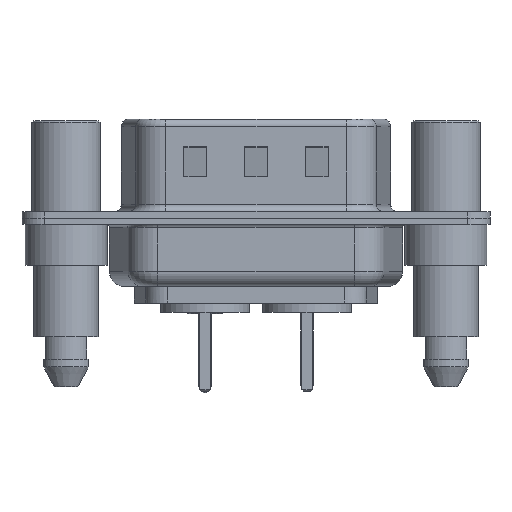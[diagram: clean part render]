
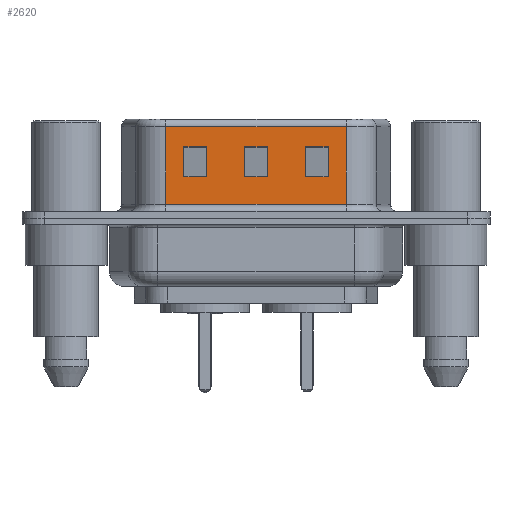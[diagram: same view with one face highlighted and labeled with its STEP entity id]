
A CAD part, front view. The second image highlights one B-rep face of the part: STEP entity #2620.
In plain terms, the highlighted planar face has unit normal (0, -1, 0).
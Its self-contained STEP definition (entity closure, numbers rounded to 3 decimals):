
#132 = LINE ( 'NONE', #7916, #21439 ) ;
#364 = DIRECTION ( 'NONE',  ( -1., 0., 0. ) ) ;
#538 = CARTESIAN_POINT ( 'NONE',  ( 18.45, -4.58, 0.9 ) ) ;
#800 = DIRECTION ( 'NONE',  ( -1., 0., 0. ) ) ;
#805 = DIRECTION ( 'NONE',  ( 0., 0., 1. ) ) ;
#951 = ORIENTED_EDGE ( 'NONE', *, *, #12862, .T. ) ;
#1283 = EDGE_LOOP ( 'NONE', ( #7963, #20948, #951, #21073 ) ) ;
#1383 = CARTESIAN_POINT ( 'NONE',  ( 7.75, -4.58, 4.705 ) ) ;
#1507 = VECTOR ( 'NONE', #8940, 1000. ) ;
#1517 = EDGE_CURVE ( 'NONE', #7936, #8701, #11608, .T. ) ;
#1711 = CARTESIAN_POINT ( 'NONE',  ( 9.25, -4.58, 6.52 ) ) ;
#2431 = VERTEX_POINT ( 'NONE', #6378 ) ;
#2462 = CARTESIAN_POINT ( 'NONE',  ( 17.25, -4.58, 4.705 ) ) ;
#2620 = ADVANCED_FACE ( 'NONE', ( #16115, #3143, #2628, #20034 ), #4380, .F. ) ;
#2628 = FACE_BOUND ( 'NONE', #5659, .T. ) ;
#2681 = CARTESIAN_POINT ( 'NONE',  ( 18.45, -4.58, 6.52 ) ) ;
#2894 = ORIENTED_EDGE ( 'NONE', *, *, #5573, .T. ) ;
#3143 = FACE_BOUND ( 'NONE', #11406, .T. ) ;
#3395 = ORIENTED_EDGE ( 'NONE', *, *, #7522, .T. ) ;
#3493 = VECTOR ( 'NONE', #6752, 1000. ) ;
#3592 = ORIENTED_EDGE ( 'NONE', *, *, #9536, .T. ) ;
#3833 = CARTESIAN_POINT ( 'NONE',  ( 22.45, -4.58, 4.705 ) ) ;
#4087 = VERTEX_POINT ( 'NONE', #10236 ) ;
#4175 = ORIENTED_EDGE ( 'NONE', *, *, #19616, .T. ) ;
#4380 = PLANE ( 'NONE',  #20349 ) ;
#4591 = VECTOR ( 'NONE', #17236, 1000. ) ;
#4650 = CARTESIAN_POINT ( 'NONE',  ( 15.75, -4.58, 4.705 ) ) ;
#4708 = LINE ( 'NONE', #6751, #13131 ) ;
#4723 = CARTESIAN_POINT ( 'NONE',  ( 7.75, -4.58, 6.52 ) ) ;
#4908 = ORIENTED_EDGE ( 'NONE', *, *, #15381, .T. ) ;
#5039 = VERTEX_POINT ( 'NONE', #21277 ) ;
#5105 = VERTEX_POINT ( 'NONE', #6813 ) ;
#5573 = EDGE_CURVE ( 'NONE', #10613, #7936, #10167, .T. ) ;
#5659 = EDGE_LOOP ( 'NONE', ( #14795, #10542, #4175, #13485 ) ) ;
#5713 = VECTOR ( 'NONE', #21201, 1000. ) ;
#5733 = DIRECTION ( 'NONE',  ( 1., 0., 0. ) ) ;
#5799 = LINE ( 'NONE', #20135, #14294 ) ;
#5944 = LINE ( 'NONE', #15727, #1507 ) ;
#6378 = CARTESIAN_POINT ( 'NONE',  ( 11.75, -4.58, 2.705 ) ) ;
#6681 = DIRECTION ( 'NONE',  ( 0., 0., -1. ) ) ;
#6751 = CARTESIAN_POINT ( 'NONE',  ( 13.25, -4.58, 6.52 ) ) ;
#6752 = DIRECTION ( 'NONE',  ( 0., 0., -1. ) ) ;
#6813 = CARTESIAN_POINT ( 'NONE',  ( 6.55, -4.58, 0.9 ) ) ;
#7059 = CARTESIAN_POINT ( 'NONE',  ( 11.75, -4.58, 6.52 ) ) ;
#7217 = VERTEX_POINT ( 'NONE', #538 ) ;
#7449 = EDGE_CURVE ( 'NONE', #5105, #7217, #132, .T. ) ;
#7522 = EDGE_CURVE ( 'NONE', #17392, #8755, #20394, .T. ) ;
#7586 = CARTESIAN_POINT ( 'NONE',  ( 18.45, -4.58, 6.52 ) ) ;
#7704 = DIRECTION ( 'NONE',  ( 1., 0., 0. ) ) ;
#7743 = DIRECTION ( 'NONE',  ( 0., 0., 1. ) ) ;
#7916 = CARTESIAN_POINT ( 'NONE',  ( 18.45, -4.58, 0.9 ) ) ;
#7936 = VERTEX_POINT ( 'NONE', #2462 ) ;
#7954 = LINE ( 'NONE', #1711, #3493 ) ;
#7963 = ORIENTED_EDGE ( 'NONE', *, *, #12365, .F. ) ;
#7995 = VECTOR ( 'NONE', #14859, 1000. ) ;
#8302 = VECTOR ( 'NONE', #7704, 1000. ) ;
#8466 = LINE ( 'NONE', #12456, #17493 ) ;
#8701 = VERTEX_POINT ( 'NONE', #14812 ) ;
#8755 = VERTEX_POINT ( 'NONE', #1383 ) ;
#8940 = DIRECTION ( 'NONE',  ( -1., 0., 0. ) ) ;
#9023 = EDGE_CURVE ( 'NONE', #2431, #15662, #11932, .T. ) ;
#9084 = VERTEX_POINT ( 'NONE', #10505 ) ;
#9168 = ORIENTED_EDGE ( 'NONE', *, *, #13507, .T. ) ;
#9296 = DIRECTION ( 'NONE',  ( 0., 0., -1. ) ) ;
#9536 = EDGE_CURVE ( 'NONE', #14445, #18924, #7954, .T. ) ;
#9953 = LINE ( 'NONE', #11099, #18441 ) ;
#10167 = LINE ( 'NONE', #3833, #5713 ) ;
#10236 = CARTESIAN_POINT ( 'NONE',  ( 18.45, -4.58, 6.02 ) ) ;
#10415 = CARTESIAN_POINT ( 'NONE',  ( 17.25, -4.58, 6.52 ) ) ;
#10505 = CARTESIAN_POINT ( 'NONE',  ( 6.55, -4.58, 6.02 ) ) ;
#10542 = ORIENTED_EDGE ( 'NONE', *, *, #19488, .T. ) ;
#10613 = VERTEX_POINT ( 'NONE', #4650 ) ;
#10643 = VECTOR ( 'NONE', #7743, 1000. ) ;
#10821 = EDGE_LOOP ( 'NONE', ( #3592, #17780, #3395, #4908 ) ) ;
#10842 = CARTESIAN_POINT ( 'NONE',  ( 22.45, -4.58, 2.705 ) ) ;
#10974 = VECTOR ( 'NONE', #364, 1000. ) ;
#11069 = EDGE_CURVE ( 'NONE', #8701, #20425, #16134, .T. ) ;
#11099 = CARTESIAN_POINT ( 'NONE',  ( 6.55, -4.58, 6.52 ) ) ;
#11396 = EDGE_CURVE ( 'NONE', #4087, #9084, #5799, .T. ) ;
#11406 = EDGE_LOOP ( 'NONE', ( #18949, #20274, #9168, #2894 ) ) ;
#11608 = LINE ( 'NONE', #10415, #15658 ) ;
#11932 = LINE ( 'NONE', #7059, #4591 ) ;
#12365 = EDGE_CURVE ( 'NONE', #4087, #7217, #13431, .T. ) ;
#12456 = CARTESIAN_POINT ( 'NONE',  ( 14.45, -4.58, 4.705 ) ) ;
#12553 = CARTESIAN_POINT ( 'NONE',  ( 15.75, -4.58, 2.705 ) ) ;
#12862 = EDGE_CURVE ( 'NONE', #9084, #5105, #9953, .T. ) ;
#13131 = VECTOR ( 'NONE', #16907, 1000. ) ;
#13431 = LINE ( 'NONE', #7586, #17423 ) ;
#13485 = ORIENTED_EDGE ( 'NONE', *, *, #9023, .T. ) ;
#13507 = EDGE_CURVE ( 'NONE', #20425, #10613, #19628, .T. ) ;
#14000 = CARTESIAN_POINT ( 'NONE',  ( 7.75, -4.58, 2.705 ) ) ;
#14008 = CARTESIAN_POINT ( 'NONE',  ( 13.25, -4.58, 2.705 ) ) ;
#14294 = VECTOR ( 'NONE', #21791, 1000. ) ;
#14445 = VERTEX_POINT ( 'NONE', #20144 ) ;
#14795 = ORIENTED_EDGE ( 'NONE', *, *, #21013, .T. ) ;
#14812 = CARTESIAN_POINT ( 'NONE',  ( 17.25, -4.58, 2.705 ) ) ;
#14859 = DIRECTION ( 'NONE',  ( 0., 0., 1. ) ) ;
#15381 = EDGE_CURVE ( 'NONE', #8755, #14445, #8466, .T. ) ;
#15390 = CARTESIAN_POINT ( 'NONE',  ( 9.25, -4.58, 2.705 ) ) ;
#15545 = LINE ( 'NONE', #18869, #10974 ) ;
#15658 = VECTOR ( 'NONE', #6681, 1000. ) ;
#15662 = VERTEX_POINT ( 'NONE', #18512 ) ;
#15727 = CARTESIAN_POINT ( 'NONE',  ( 14.45, -4.58, 2.705 ) ) ;
#16115 = FACE_BOUND ( 'NONE', #10821, .T. ) ;
#16134 = LINE ( 'NONE', #10842, #20054 ) ;
#16170 = CARTESIAN_POINT ( 'NONE',  ( 18.45, -4.58, 4.705 ) ) ;
#16250 = DIRECTION ( 'NONE',  ( 0., 0., -1. ) ) ;
#16907 = DIRECTION ( 'NONE',  ( 0., 0., -1. ) ) ;
#17236 = DIRECTION ( 'NONE',  ( 0., 0., 1. ) ) ;
#17392 = VERTEX_POINT ( 'NONE', #14000 ) ;
#17423 = VECTOR ( 'NONE', #9296, 1000. ) ;
#17493 = VECTOR ( 'NONE', #5733, 1000. ) ;
#17780 = ORIENTED_EDGE ( 'NONE', *, *, #21677, .T. ) ;
#17910 = CARTESIAN_POINT ( 'NONE',  ( 15.75, -4.58, 6.52 ) ) ;
#18441 = VECTOR ( 'NONE', #16250, 1000. ) ;
#18512 = CARTESIAN_POINT ( 'NONE',  ( 11.75, -4.58, 4.705 ) ) ;
#18869 = CARTESIAN_POINT ( 'NONE',  ( 18.45, -4.58, 2.705 ) ) ;
#18924 = VERTEX_POINT ( 'NONE', #15390 ) ;
#18949 = ORIENTED_EDGE ( 'NONE', *, *, #1517, .T. ) ;
#19488 = EDGE_CURVE ( 'NONE', #5039, #21674, #4708, .T. ) ;
#19616 = EDGE_CURVE ( 'NONE', #21674, #2431, #15545, .T. ) ;
#19628 = LINE ( 'NONE', #17910, #10643 ) ;
#19733 = DIRECTION ( 'NONE',  ( 1., 0., 0. ) ) ;
#19834 = DIRECTION ( 'NONE',  ( 0., 1., 0. ) ) ;
#20034 = FACE_OUTER_BOUND ( 'NONE', #1283, .T. ) ;
#20054 = VECTOR ( 'NONE', #800, 1000. ) ;
#20135 = CARTESIAN_POINT ( 'NONE',  ( 18.45, -4.58, 6.02 ) ) ;
#20144 = CARTESIAN_POINT ( 'NONE',  ( 9.25, -4.58, 4.705 ) ) ;
#20274 = ORIENTED_EDGE ( 'NONE', *, *, #11069, .T. ) ;
#20349 = AXIS2_PLACEMENT_3D ( 'NONE', #2681, #19834, #805 ) ;
#20394 = LINE ( 'NONE', #4723, #7995 ) ;
#20425 = VERTEX_POINT ( 'NONE', #12553 ) ;
#20948 = ORIENTED_EDGE ( 'NONE', *, *, #11396, .T. ) ;
#21013 = EDGE_CURVE ( 'NONE', #15662, #5039, #21727, .T. ) ;
#21073 = ORIENTED_EDGE ( 'NONE', *, *, #7449, .T. ) ;
#21201 = DIRECTION ( 'NONE',  ( 1., 0., 0. ) ) ;
#21277 = CARTESIAN_POINT ( 'NONE',  ( 13.25, -4.58, 4.705 ) ) ;
#21439 = VECTOR ( 'NONE', #19733, 1000. ) ;
#21674 = VERTEX_POINT ( 'NONE', #14008 ) ;
#21677 = EDGE_CURVE ( 'NONE', #18924, #17392, #5944, .T. ) ;
#21727 = LINE ( 'NONE', #16170, #8302 ) ;
#21791 = DIRECTION ( 'NONE',  ( -1., 0., 0. ) ) ;
